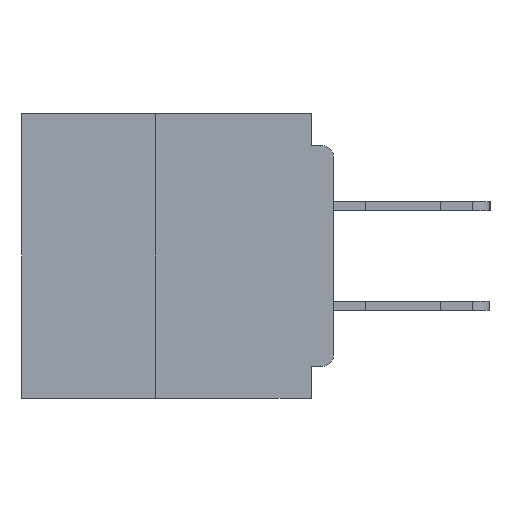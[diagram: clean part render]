
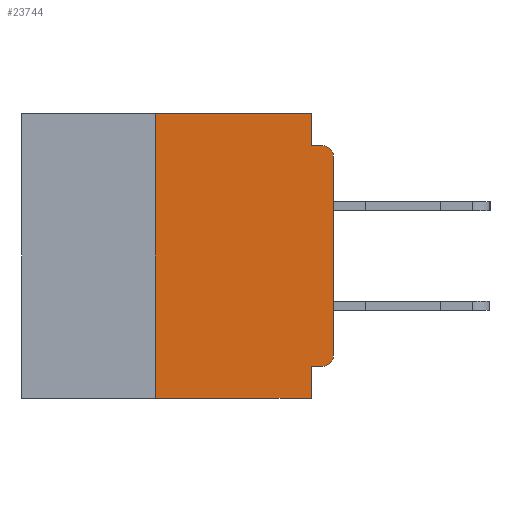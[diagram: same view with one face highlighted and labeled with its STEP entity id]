
A CAD part, left-side view. The second image highlights one B-rep face of the part: STEP entity #23744.
In plain terms, the highlighted planar face has unit normal (-1, 0, 0).
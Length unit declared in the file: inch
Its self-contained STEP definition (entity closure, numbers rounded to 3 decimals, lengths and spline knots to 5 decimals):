
#229 = AXIS2_PLACEMENT_3D ( 'NONE', #6120, #33072, #9985 ) ;
#616 = ORIENTED_EDGE ( 'NONE', *, *, #25684, .F. ) ;
#1479 = EDGE_CURVE ( 'NONE', #35355, #3732, #13909, .T. ) ;
#2330 = LINE ( 'NONE', #44047, #49875 ) ;
#2474 = CIRCLE ( 'NONE', #20696, 0.015 ) ;
#3732 = VERTEX_POINT ( 'NONE', #14190 ) ;
#4544 = LINE ( 'NONE', #22117, #14760 ) ;
#4980 = LINE ( 'NONE', #8538, #13968 ) ;
#5043 = EDGE_CURVE ( 'NONE', #9775, #28718, #41596, .T. ) ;
#6120 = CARTESIAN_POINT ( 'NONE',  ( 0., 0.437, 0. ) ) ;
#6399 = ORIENTED_EDGE ( 'NONE', *, *, #21778, .F. ) ;
#7023 = DIRECTION ( 'NONE',  ( 0., -1., 0. ) ) ;
#7051 = DIRECTION ( 'NONE',  ( 0., 1., 0. ) ) ;
#7526 = CIRCLE ( 'NONE', #19188, 0.015 ) ;
#8538 = CARTESIAN_POINT ( 'NONE',  ( 0., 0.437, 0. ) ) ;
#8568 = VECTOR ( 'NONE', #32440, 39.37008 ) ;
#8895 = ORIENTED_EDGE ( 'NONE', *, *, #46926, .F. ) ;
#9423 = CARTESIAN_POINT ( 'NONE',  ( 0., 0.031, 0. ) ) ;
#9775 = VERTEX_POINT ( 'NONE', #16851 ) ;
#9985 = DIRECTION ( 'NONE',  ( 0., 0., -1. ) ) ;
#11029 = ORIENTED_EDGE ( 'NONE', *, *, #44373, .T. ) ;
#11840 = DIRECTION ( 'NONE',  ( -1., 0., 0. ) ) ;
#12429 = DIRECTION ( 'NONE',  ( 0., -1., 0. ) ) ;
#12532 = CARTESIAN_POINT ( 'NONE',  ( 0., 0.031, -0.355 ) ) ;
#12903 = LINE ( 'NONE', #30094, #14099 ) ;
#13909 = LINE ( 'NONE', #35732, #30829 ) ;
#13968 = VECTOR ( 'NONE', #12429, 39.37008 ) ;
#13995 = ORIENTED_EDGE ( 'NONE', *, *, #31806, .T. ) ;
#14042 = ORIENTED_EDGE ( 'NONE', *, *, #36999, .T. ) ;
#14099 = VECTOR ( 'NONE', #7023, 39.37008 ) ;
#14190 = CARTESIAN_POINT ( 'NONE',  ( 0., 0., -0.06 ) ) ;
#14760 = VECTOR ( 'NONE', #29865, 39.37008 ) ;
#15735 = CARTESIAN_POINT ( 'NONE',  ( 0., 0.25, -0.4 ) ) ;
#16851 = CARTESIAN_POINT ( 'NONE',  ( 0., 0.015, -0.355 ) ) ;
#16923 = CARTESIAN_POINT ( 'NONE',  ( 0., 0.25, -0.4 ) ) ;
#17606 = VERTEX_POINT ( 'NONE', #41477 ) ;
#19188 = AXIS2_PLACEMENT_3D ( 'NONE', #34913, #11840, #38802 ) ;
#19290 = VERTEX_POINT ( 'NONE', #47515 ) ;
#19722 = ORIENTED_EDGE ( 'NONE', *, *, #5043, .F. ) ;
#20403 = DIRECTION ( 'NONE',  ( 0., 0., 1. ) ) ;
#20680 = DIRECTION ( 'NONE',  ( -1., 0., 0. ) ) ;
#20696 = AXIS2_PLACEMENT_3D ( 'NONE', #43753, #20680, #47584 ) ;
#21778 = EDGE_CURVE ( 'NONE', #19290, #17606, #4980, .T. ) ;
#22117 = CARTESIAN_POINT ( 'NONE',  ( 0., 0., -0.045 ) ) ;
#22356 = CARTESIAN_POINT ( 'NONE',  ( 0., 0., -0.355 ) ) ;
#22360 = VERTEX_POINT ( 'NONE', #15735 ) ;
#23204 = CARTESIAN_POINT ( 'NONE',  ( 0., 0.031, -0.4 ) ) ;
#23744 = ADVANCED_FACE ( 'NONE', ( #34901 ), #36787, .F. ) ;
#24583 = LINE ( 'NONE', #9423, #33639 ) ;
#24932 = CARTESIAN_POINT ( 'NONE',  ( 0., 0.031, -0.045 ) ) ;
#25684 = EDGE_CURVE ( 'NONE', #40454, #37310, #4544, .T. ) ;
#28718 = VERTEX_POINT ( 'NONE', #12532 ) ;
#28863 = EDGE_CURVE ( 'NONE', #28718, #30621, #2330, .T. ) ;
#29865 = DIRECTION ( 'NONE',  ( 0., -1., 0. ) ) ;
#30094 = CARTESIAN_POINT ( 'NONE',  ( 0., 0.437, -0.4 ) ) ;
#30621 = VERTEX_POINT ( 'NONE', #23204 ) ;
#30829 = VECTOR ( 'NONE', #20403, 39.37008 ) ;
#31806 = EDGE_CURVE ( 'NONE', #9775, #35355, #7526, .T. ) ;
#32440 = DIRECTION ( 'NONE',  ( 0., 0., 1. ) ) ;
#33072 = DIRECTION ( 'NONE',  ( 1., 0., 0. ) ) ;
#33639 = VECTOR ( 'NONE', #44137, 39.37008 ) ;
#33747 = ORIENTED_EDGE ( 'NONE', *, *, #1479, .T. ) ;
#34901 = FACE_OUTER_BOUND ( 'NONE', #37341, .T. ) ;
#34913 = CARTESIAN_POINT ( 'NONE',  ( 0., 0.015, -0.34 ) ) ;
#35355 = VERTEX_POINT ( 'NONE', #37006 ) ;
#35732 = CARTESIAN_POINT ( 'NONE',  ( 0., 0., 0. ) ) ;
#36787 = PLANE ( 'NONE',  #229 ) ;
#36999 = EDGE_CURVE ( 'NONE', #3732, #37310, #2474, .T. ) ;
#37006 = CARTESIAN_POINT ( 'NONE',  ( 0., 0., -0.34 ) ) ;
#37310 = VERTEX_POINT ( 'NONE', #38007 ) ;
#37341 = EDGE_LOOP ( 'NONE', ( #33747, #14042, #616, #47862, #6399, #8895, #11029, #40128, #19722, #13995 ) ) ;
#38007 = CARTESIAN_POINT ( 'NONE',  ( 0., 0.015, -0.045 ) ) ;
#38802 = DIRECTION ( 'NONE',  ( 0., 0., -1. ) ) ;
#39188 = VECTOR ( 'NONE', #7051, 39.37008 ) ;
#40128 = ORIENTED_EDGE ( 'NONE', *, *, #28863, .F. ) ;
#40454 = VERTEX_POINT ( 'NONE', #24932 ) ;
#40546 = LINE ( 'NONE', #16923, #8568 ) ;
#41477 = CARTESIAN_POINT ( 'NONE',  ( 0., 0.031, 0. ) ) ;
#41596 = LINE ( 'NONE', #22356, #39188 ) ;
#43753 = CARTESIAN_POINT ( 'NONE',  ( 0., 0.015, -0.06 ) ) ;
#44047 = CARTESIAN_POINT ( 'NONE',  ( 0., 0.031, -0.4 ) ) ;
#44137 = DIRECTION ( 'NONE',  ( 0., 0., -1. ) ) ;
#44373 = EDGE_CURVE ( 'NONE', #22360, #30621, #12903, .T. ) ;
#46926 = EDGE_CURVE ( 'NONE', #22360, #19290, #40546, .T. ) ;
#47515 = CARTESIAN_POINT ( 'NONE',  ( 0., 0.25, 0. ) ) ;
#47584 = DIRECTION ( 'NONE',  ( 0., 0., -1. ) ) ;
#47849 = DIRECTION ( 'NONE',  ( 0., 0., -1. ) ) ;
#47862 = ORIENTED_EDGE ( 'NONE', *, *, #49455, .F. ) ;
#49455 = EDGE_CURVE ( 'NONE', #17606, #40454, #24583, .T. ) ;
#49875 = VECTOR ( 'NONE', #47849, 39.37008 ) ;
